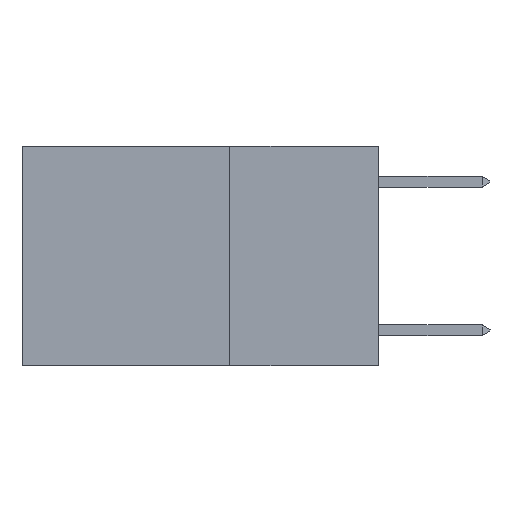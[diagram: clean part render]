
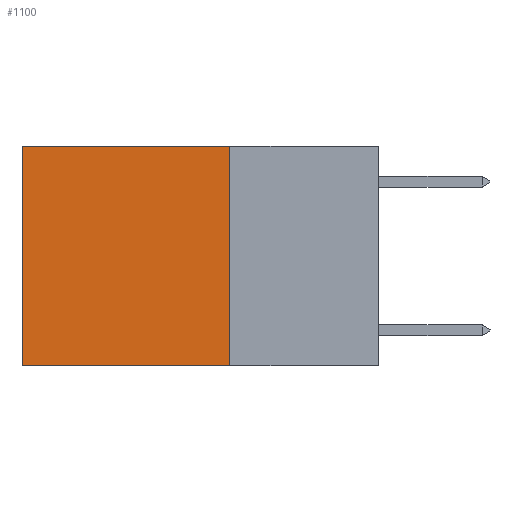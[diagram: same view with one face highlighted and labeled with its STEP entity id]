
A CAD part, left-side view. The second image highlights one B-rep face of the part: STEP entity #1100.
In plain terms, the highlighted planar face has unit normal (-1, 0, 0).
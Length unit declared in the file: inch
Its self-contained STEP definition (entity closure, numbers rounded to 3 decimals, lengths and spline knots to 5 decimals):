
#329 = FACE_OUTER_BOUND ( 'NONE', #16576, .T. ) ;
#1100 = ADVANCED_FACE ( 'NONE', ( #329 ), #18920, .F. ) ;
#1898 = DIRECTION ( 'NONE',  ( 0., 1., 0. ) ) ;
#2636 = VERTEX_POINT ( 'NONE', #3867 ) ;
#3867 = CARTESIAN_POINT ( 'NONE',  ( 0.2625, 0.25, 0. ) ) ;
#4049 = CARTESIAN_POINT ( 'NONE',  ( 0.2625, 0.25, -0.37 ) ) ;
#4348 = DIRECTION ( 'NONE',  ( 0., 1., 0. ) ) ;
#4688 = ORIENTED_EDGE ( 'NONE', *, *, #11645, .F. ) ;
#6617 = ORIENTED_EDGE ( 'NONE', *, *, #16963, .T. ) ;
#6761 = ORIENTED_EDGE ( 'NONE', *, *, #19716, .T. ) ;
#7437 = ORIENTED_EDGE ( 'NONE', *, *, #17286, .F. ) ;
#11645 = EDGE_CURVE ( 'NONE', #12536, #26435, #22120, .T. ) ;
#12536 = VERTEX_POINT ( 'NONE', #13574 ) ;
#13574 = CARTESIAN_POINT ( 'NONE',  ( 0.2625, 0.25, -0.37 ) ) ;
#14002 = CARTESIAN_POINT ( 'NONE',  ( 0.2625, 0.6, 0. ) ) ;
#16291 = DIRECTION ( 'NONE',  ( 0., 0., -1. ) ) ;
#16442 = DIRECTION ( 'NONE',  ( 0., 0., -1. ) ) ;
#16576 = EDGE_LOOP ( 'NONE', ( #6761, #4688, #7437, #6617 ) ) ;
#16645 = CARTESIAN_POINT ( 'NONE',  ( 0.2625, 0.25, 0. ) ) ;
#16963 = EDGE_CURVE ( 'NONE', #2636, #25921, #20297, .T. ) ;
#17286 = EDGE_CURVE ( 'NONE', #2636, #12536, #17875, .T. ) ;
#17875 = LINE ( 'NONE', #16645, #18084 ) ;
#18084 = VECTOR ( 'NONE', #16442, 39.37008 ) ;
#18488 = VECTOR ( 'NONE', #4348, 39.37008 ) ;
#18522 = DIRECTION ( 'NONE',  ( 0., 0., -1. ) ) ;
#18564 = DIRECTION ( 'NONE',  ( 1., 0., 0. ) ) ;
#18580 = CARTESIAN_POINT ( 'NONE',  ( 0.2625, 0.6, 0. ) ) ;
#18806 = CARTESIAN_POINT ( 'NONE',  ( 0.2625, 0.25, 0. ) ) ;
#18920 = PLANE ( 'NONE',  #24294 ) ;
#19716 = EDGE_CURVE ( 'NONE', #25921, #26435, #26203, .T. ) ;
#20297 = LINE ( 'NONE', #28132, #20356 ) ;
#20356 = VECTOR ( 'NONE', #1898, 39.37008 ) ;
#22120 = LINE ( 'NONE', #4049, #18488 ) ;
#24294 = AXIS2_PLACEMENT_3D ( 'NONE', #18806, #18564, #18522 ) ;
#25574 = VECTOR ( 'NONE', #16291, 39.37008 ) ;
#25921 = VERTEX_POINT ( 'NONE', #18580 ) ;
#26203 = LINE ( 'NONE', #14002, #25574 ) ;
#26435 = VERTEX_POINT ( 'NONE', #27474 ) ;
#27474 = CARTESIAN_POINT ( 'NONE',  ( 0.2625, 0.6, -0.37 ) ) ;
#28132 = CARTESIAN_POINT ( 'NONE',  ( 0.2625, 0.25, 0. ) ) ;
